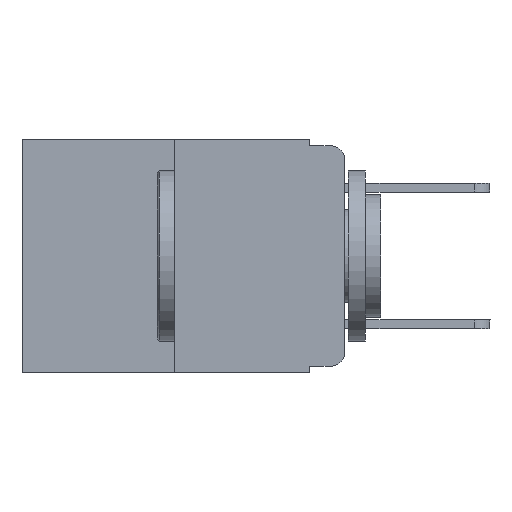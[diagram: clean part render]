
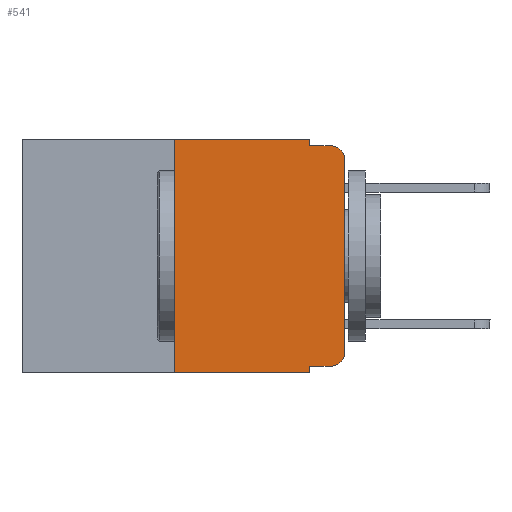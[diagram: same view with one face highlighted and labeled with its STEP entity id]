
A CAD part, left-side view. The second image highlights one B-rep face of the part: STEP entity #541.
In plain terms, the highlighted planar face has unit normal (-1, 0, 0).
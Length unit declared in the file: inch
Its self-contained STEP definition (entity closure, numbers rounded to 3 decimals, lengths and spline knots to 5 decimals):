
#140 = DIRECTION ( 'NONE',  ( 0., -1., 0. ) ) ;
#216 = CARTESIAN_POINT ( 'NONE',  ( 0., 0.051, -0.343 ) ) ;
#222 = CARTESIAN_POINT ( 'NONE',  ( 0., 0.051, -0.01 ) ) ;
#339 = LINE ( 'NONE', #7053, #8873 ) ;
#386 = EDGE_CURVE ( 'NONE', #17665, #12253, #15220, .T. ) ;
#541 = ADVANCED_FACE ( 'NONE', ( #4345 ), #18792, .F. ) ;
#769 = CARTESIAN_POINT ( 'NONE',  ( 0., 0., 0. ) ) ;
#994 = VERTEX_POINT ( 'NONE', #2208 ) ;
#1522 = ORIENTED_EDGE ( 'NONE', *, *, #4730, .F. ) ;
#1747 = CARTESIAN_POINT ( 'NONE',  ( 0., 0.02, -0.313 ) ) ;
#2192 = DIRECTION ( 'NONE',  ( 0., 0., -1. ) ) ;
#2208 = CARTESIAN_POINT ( 'NONE',  ( 0., 0.25, -0.343 ) ) ;
#2620 = VECTOR ( 'NONE', #20814, 39.37008 ) ;
#2982 = CARTESIAN_POINT ( 'NONE',  ( 0., 0.02, -0.03 ) ) ;
#3170 = VECTOR ( 'NONE', #4255, 39.37008 ) ;
#3663 = VERTEX_POINT ( 'NONE', #12587 ) ;
#4255 = DIRECTION ( 'NONE',  ( 0., 0., -1. ) ) ;
#4256 = VERTEX_POINT ( 'NONE', #20674 ) ;
#4345 = FACE_OUTER_BOUND ( 'NONE', #13022, .T. ) ;
#4470 = EDGE_CURVE ( 'NONE', #13815, #17161, #339, .T. ) ;
#4476 = ORIENTED_EDGE ( 'NONE', *, *, #9829, .F. ) ;
#4606 = LINE ( 'NONE', #8890, #13654 ) ;
#4730 = EDGE_CURVE ( 'NONE', #19498, #16065, #20618, .T. ) ;
#4805 = DIRECTION ( 'NONE',  ( -1., 0., 0. ) ) ;
#5103 = ORIENTED_EDGE ( 'NONE', *, *, #6423, .T. ) ;
#5276 = DIRECTION ( 'NONE',  ( 0., 0., -1. ) ) ;
#5652 = ORIENTED_EDGE ( 'NONE', *, *, #8197, .F. ) ;
#5702 = CARTESIAN_POINT ( 'NONE',  ( 0., 0.051, 0. ) ) ;
#5767 = LINE ( 'NONE', #769, #11721 ) ;
#6423 = EDGE_CURVE ( 'NONE', #13815, #4256, #13738, .T. ) ;
#6586 = ORIENTED_EDGE ( 'NONE', *, *, #11216, .F. ) ;
#6599 = LINE ( 'NONE', #222, #19159 ) ;
#6659 = DIRECTION ( 'NONE',  ( 0., 0., -1. ) ) ;
#6851 = EDGE_CURVE ( 'NONE', #994, #17161, #6962, .T. ) ;
#6962 = LINE ( 'NONE', #14313, #19006 ) ;
#7053 = CARTESIAN_POINT ( 'NONE',  ( 0., 0.051, 0. ) ) ;
#7092 = VECTOR ( 'NONE', #11264, 39.37008 ) ;
#7270 = DIRECTION ( 'NONE',  ( 0., 0., 1. ) ) ;
#7376 = ORIENTED_EDGE ( 'NONE', *, *, #4470, .F. ) ;
#8197 = EDGE_CURVE ( 'NONE', #994, #16786, #4606, .T. ) ;
#8782 = CARTESIAN_POINT ( 'NONE',  ( 0., 0.473, 0. ) ) ;
#8873 = VECTOR ( 'NONE', #5276, 39.37008 ) ;
#8890 = CARTESIAN_POINT ( 'NONE',  ( 0., 0.25, 0. ) ) ;
#9451 = AXIS2_PLACEMENT_3D ( 'NONE', #1747, #4805, #6659 ) ;
#9586 = CARTESIAN_POINT ( 'NONE',  ( 0., 0.473, 0. ) ) ;
#9742 = DIRECTION ( 'NONE',  ( -1., 0., 0. ) ) ;
#9829 = EDGE_CURVE ( 'NONE', #16786, #19498, #14884, .T. ) ;
#10594 = DIRECTION ( 'NONE',  ( 0., 0., 1. ) ) ;
#10651 = ORIENTED_EDGE ( 'NONE', *, *, #21404, .T. ) ;
#10980 = DIRECTION ( 'NONE',  ( 0., -1., 0. ) ) ;
#11216 = EDGE_CURVE ( 'NONE', #16065, #12253, #6599, .T. ) ;
#11264 = DIRECTION ( 'NONE',  ( 0., -1., 0. ) ) ;
#11721 = VECTOR ( 'NONE', #7270, 39.37008 ) ;
#12253 = VERTEX_POINT ( 'NONE', #14721 ) ;
#12411 = CARTESIAN_POINT ( 'NONE',  ( 0., 0.051, -0.333 ) ) ;
#12587 = CARTESIAN_POINT ( 'NONE',  ( 0., 0., -0.313 ) ) ;
#13022 = EDGE_LOOP ( 'NONE', ( #10651, #19584, #6586, #1522, #4476, #5652, #19871, #7376, #5103, #15933 ) ) ;
#13518 = CARTESIAN_POINT ( 'NONE',  ( 0., 0.051, 0. ) ) ;
#13654 = VECTOR ( 'NONE', #10594, 39.37008 ) ;
#13738 = LINE ( 'NONE', #12411, #2620 ) ;
#13815 = VERTEX_POINT ( 'NONE', #15653 ) ;
#14313 = CARTESIAN_POINT ( 'NONE',  ( 0., 0.473, -0.343 ) ) ;
#14596 = CARTESIAN_POINT ( 'NONE',  ( 0., 0., -0.03 ) ) ;
#14721 = CARTESIAN_POINT ( 'NONE',  ( 0., 0.02, -0.01 ) ) ;
#14884 = LINE ( 'NONE', #9586, #7092 ) ;
#15053 = AXIS2_PLACEMENT_3D ( 'NONE', #8782, #15310, #2192 ) ;
#15170 = CARTESIAN_POINT ( 'NONE',  ( 0., 0.051, -0.01 ) ) ;
#15220 = CIRCLE ( 'NONE', #18459, 0.02 ) ;
#15310 = DIRECTION ( 'NONE',  ( 1., 0., 0. ) ) ;
#15653 = CARTESIAN_POINT ( 'NONE',  ( 0., 0.051, -0.333 ) ) ;
#15933 = ORIENTED_EDGE ( 'NONE', *, *, #18313, .T. ) ;
#16065 = VERTEX_POINT ( 'NONE', #15170 ) ;
#16522 = CIRCLE ( 'NONE', #9451, 0.02 ) ;
#16786 = VERTEX_POINT ( 'NONE', #17533 ) ;
#17161 = VERTEX_POINT ( 'NONE', #216 ) ;
#17533 = CARTESIAN_POINT ( 'NONE',  ( 0., 0.25, 0. ) ) ;
#17665 = VERTEX_POINT ( 'NONE', #14596 ) ;
#18313 = EDGE_CURVE ( 'NONE', #4256, #3663, #16522, .T. ) ;
#18459 = AXIS2_PLACEMENT_3D ( 'NONE', #2982, #9742, #19851 ) ;
#18792 = PLANE ( 'NONE',  #15053 ) ;
#19006 = VECTOR ( 'NONE', #10980, 39.37008 ) ;
#19159 = VECTOR ( 'NONE', #140, 39.37008 ) ;
#19498 = VERTEX_POINT ( 'NONE', #13518 ) ;
#19584 = ORIENTED_EDGE ( 'NONE', *, *, #386, .T. ) ;
#19851 = DIRECTION ( 'NONE',  ( 0., 0., -1. ) ) ;
#19871 = ORIENTED_EDGE ( 'NONE', *, *, #6851, .T. ) ;
#20618 = LINE ( 'NONE', #5702, #3170 ) ;
#20674 = CARTESIAN_POINT ( 'NONE',  ( 0., 0.02, -0.333 ) ) ;
#20814 = DIRECTION ( 'NONE',  ( 0., -1., 0. ) ) ;
#21404 = EDGE_CURVE ( 'NONE', #3663, #17665, #5767, .T. ) ;
